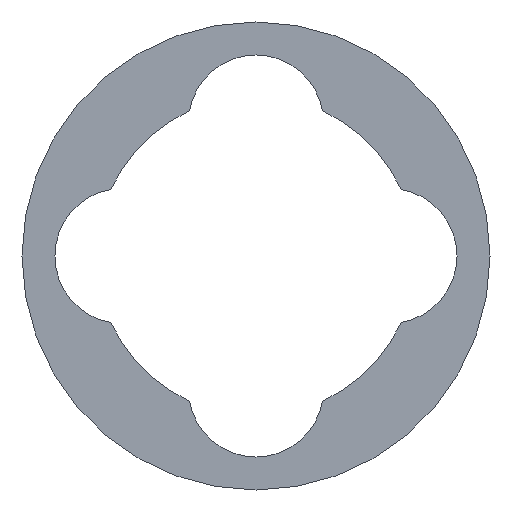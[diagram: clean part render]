
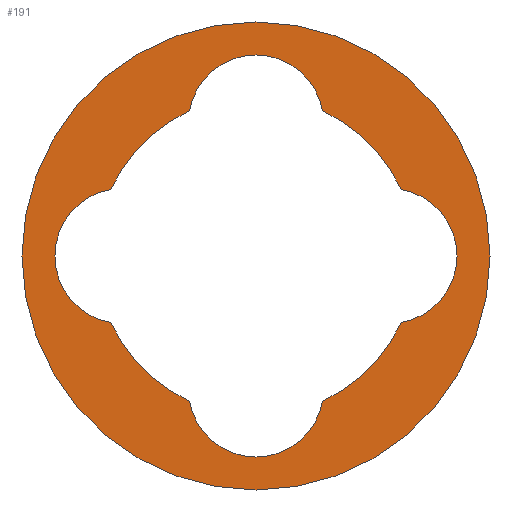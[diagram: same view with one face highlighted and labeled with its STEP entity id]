
A CAD part, front view. The second image highlights one B-rep face of the part: STEP entity #191.
In plain terms, the highlighted planar face has unit normal (0, -1, 0).
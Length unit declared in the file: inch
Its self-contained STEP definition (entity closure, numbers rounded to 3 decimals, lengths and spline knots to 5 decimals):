
#15=FACE_BOUND('',#35,.T.);
#17=PLANE('',#230);
#23=FACE_OUTER_BOUND('',#34,.T.);
#34=EDGE_LOOP('',(#140));
#35=EDGE_LOOP('',(#141,#142,#143,#144,#145,#146,#147,#148));
#61=CIRCLE('',#219,0.11821);
#63=CIRCLE('',#222,0.11821);
#65=CIRCLE('',#225,0.11821);
#67=CIRCLE('',#228,0.11821);
#69=CIRCLE('',#231,0.17323);
#70=CIRCLE('',#232,0.05);
#71=CIRCLE('',#233,0.05);
#72=CIRCLE('',#234,0.05);
#73=CIRCLE('',#235,0.05);
#79=VERTEX_POINT('',#318);
#80=VERTEX_POINT('',#319);
#83=VERTEX_POINT('',#327);
#84=VERTEX_POINT('',#328);
#87=VERTEX_POINT('',#336);
#88=VERTEX_POINT('',#337);
#91=VERTEX_POINT('',#345);
#92=VERTEX_POINT('',#346);
#95=VERTEX_POINT('',#354);
#97=EDGE_CURVE('',#79,#80,#61,.T.);
#101=EDGE_CURVE('',#83,#84,#63,.T.);
#105=EDGE_CURVE('',#87,#88,#65,.T.);
#109=EDGE_CURVE('',#91,#92,#67,.T.);
#113=EDGE_CURVE('',#95,#95,#69,.T.);
#114=EDGE_CURVE('',#79,#88,#70,.T.);
#115=EDGE_CURVE('',#91,#80,#71,.T.);
#116=EDGE_CURVE('',#83,#92,#72,.T.);
#117=EDGE_CURVE('',#84,#87,#73,.T.);
#140=ORIENTED_EDGE('',*,*,#113,.F.);
#141=ORIENTED_EDGE('',*,*,#114,.F.);
#142=ORIENTED_EDGE('',*,*,#97,.T.);
#143=ORIENTED_EDGE('',*,*,#115,.F.);
#144=ORIENTED_EDGE('',*,*,#109,.T.);
#145=ORIENTED_EDGE('',*,*,#116,.F.);
#146=ORIENTED_EDGE('',*,*,#101,.T.);
#147=ORIENTED_EDGE('',*,*,#117,.T.);
#148=ORIENTED_EDGE('',*,*,#105,.T.);
#191=ADVANCED_FACE('',(#23,#15),#17,.F.);
#219=AXIS2_PLACEMENT_3D('',#320,#251,#252);
#222=AXIS2_PLACEMENT_3D('',#329,#259,#260);
#225=AXIS2_PLACEMENT_3D('',#338,#267,#268);
#228=AXIS2_PLACEMENT_3D('',#347,#275,#276);
#230=AXIS2_PLACEMENT_3D('',#353,#281,#282);
#231=AXIS2_PLACEMENT_3D('',#355,#283,#284);
#232=AXIS2_PLACEMENT_3D('',#356,#285,#286);
#233=AXIS2_PLACEMENT_3D('',#357,#287,#288);
#234=AXIS2_PLACEMENT_3D('',#358,#289,#290);
#235=AXIS2_PLACEMENT_3D('',#359,#291,#292);
#251=DIRECTION('center_axis',(0.,1.,0.));
#252=DIRECTION('ref_axis',(-1.,0.,0.));
#259=DIRECTION('center_axis',(0.,1.,0.));
#260=DIRECTION('ref_axis',(-1.,0.,0.));
#267=DIRECTION('center_axis',(0.,1.,0.));
#268=DIRECTION('ref_axis',(-1.,0.,0.));
#275=DIRECTION('center_axis',(0.,1.,0.));
#276=DIRECTION('ref_axis',(-1.,0.,0.));
#281=DIRECTION('center_axis',(0.,1.,0.));
#282=DIRECTION('ref_axis',(0.,0.,1.));
#283=DIRECTION('center_axis',(0.,1.,0.));
#284=DIRECTION('ref_axis',(-1.,0.,0.));
#285=DIRECTION('center_axis',(0.,-1.,0.));
#286=DIRECTION('ref_axis',(-1.,0.,0.));
#287=DIRECTION('center_axis',(0.,-1.,0.));
#288=DIRECTION('ref_axis',(-1.,0.,0.));
#289=DIRECTION('center_axis',(0.,-1.,0.));
#290=DIRECTION('ref_axis',(-1.,0.,0.));
#291=DIRECTION('center_axis',(0.,1.,0.));
#292=DIRECTION('ref_axis',(0.172,0.,0.985));
#318=CARTESIAN_POINT('',(0.04925,1.,0.10746));
#319=CARTESIAN_POINT('',(0.10746,1.,0.04925));
#320=CARTESIAN_POINT('Origin',(0.,1.,0.));
#327=CARTESIAN_POINT('',(-0.04925,1.,-0.10746));
#328=CARTESIAN_POINT('',(-0.10746,1.,-0.04926));
#329=CARTESIAN_POINT('Origin',(0.,1.,0.));
#336=CARTESIAN_POINT('',(-0.10746,1.,0.04926));
#337=CARTESIAN_POINT('',(-0.04925,1.,0.10746));
#338=CARTESIAN_POINT('Origin',(0.,1.,0.));
#345=CARTESIAN_POINT('',(0.10746,1.,-0.04925));
#346=CARTESIAN_POINT('',(0.04925,1.,-0.10746));
#347=CARTESIAN_POINT('Origin',(0.,1.,0.));
#353=CARTESIAN_POINT('Origin',(0.,1.,0.));
#354=CARTESIAN_POINT('',(0.17323,1.,0.));
#355=CARTESIAN_POINT('Origin',(0.,1.,0.));
#356=CARTESIAN_POINT('Origin',(0.,1.,0.09881));
#357=CARTESIAN_POINT('Origin',(0.09881,1.,0.));
#358=CARTESIAN_POINT('Origin',(0.,1.,-0.09881));
#359=CARTESIAN_POINT('Origin',(-0.09887,1.,0.));
